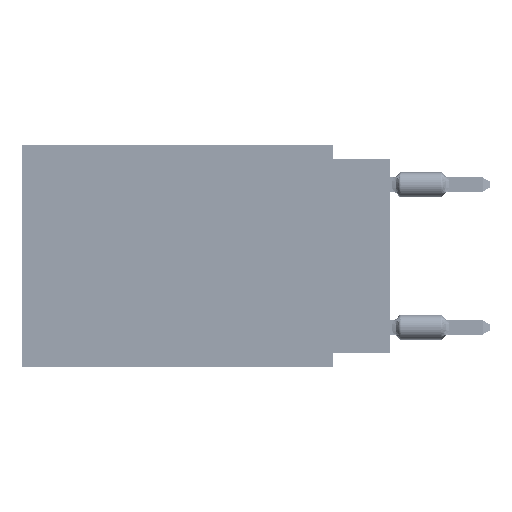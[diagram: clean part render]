
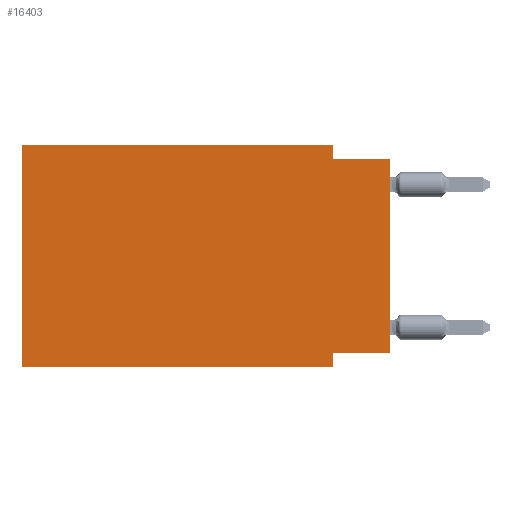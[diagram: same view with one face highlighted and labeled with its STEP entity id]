
A CAD part, left-side view. The second image highlights one B-rep face of the part: STEP entity #16403.
In plain terms, the highlighted planar face has unit normal (-1, 0, 0).
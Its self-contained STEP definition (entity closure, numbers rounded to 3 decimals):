
#2498 = PLANE ( 'NONE',  #29205 ) ;
#3460 = CARTESIAN_POINT ( 'NONE',  ( 0., 16.383, 0. ) ) ;
#4499 = DIRECTION ( 'NONE',  ( 0., 0., 1. ) ) ;
#5899 = ORIENTED_EDGE ( 'NONE', *, *, #72628, .F. ) ;
#9023 = CARTESIAN_POINT ( 'NONE',  ( 0., 16.383, 0. ) ) ;
#9397 = CARTESIAN_POINT ( 'NONE',  ( 0., 16.383, -9.906 ) ) ;
#9549 = VECTOR ( 'NONE', #66764, 1000. ) ;
#11398 = EDGE_CURVE ( 'NONE', #43634, #59774, #83114, .T. ) ;
#12213 = CARTESIAN_POINT ( 'NONE',  ( 0., 2.54, -0.635 ) ) ;
#13168 = VERTEX_POINT ( 'NONE', #40027 ) ;
#15576 = CARTESIAN_POINT ( 'NONE',  ( 0., 16.383, 0. ) ) ;
#15916 = LINE ( 'NONE', #9397, #35079 ) ;
#16403 = ADVANCED_FACE ( 'NONE', ( #55462 ), #2498, .F. ) ;
#19029 = LINE ( 'NONE', #39016, #73294 ) ;
#19997 = VECTOR ( 'NONE', #4499, 1000. ) ;
#20583 = DIRECTION ( 'NONE',  ( 0., 0., -1. ) ) ;
#21373 = VECTOR ( 'NONE', #48585, 1000. ) ;
#24513 = VERTEX_POINT ( 'NONE', #62157 ) ;
#25039 = CARTESIAN_POINT ( 'NONE',  ( 0., 0., -9.271 ) ) ;
#25801 = LINE ( 'NONE', #33173, #53826 ) ;
#26759 = EDGE_CURVE ( 'NONE', #47627, #76217, #25801, .T. ) ;
#27431 = ORIENTED_EDGE ( 'NONE', *, *, #43251, .F. ) ;
#29205 = AXIS2_PLACEMENT_3D ( 'NONE', #9023, #81532, #74999 ) ;
#29283 = VECTOR ( 'NONE', #32842, 1000. ) ;
#30302 = VERTEX_POINT ( 'NONE', #3460 ) ;
#30586 = VECTOR ( 'NONE', #82676, 1000. ) ;
#32842 = DIRECTION ( 'NONE',  ( 0., 1., 0. ) ) ;
#33161 = EDGE_CURVE ( 'NONE', #43634, #47627, #64108, .T. ) ;
#33173 = CARTESIAN_POINT ( 'NONE',  ( 0., 2.54, -9.906 ) ) ;
#34630 = LINE ( 'NONE', #47665, #9549 ) ;
#35079 = VECTOR ( 'NONE', #49338, 1000. ) ;
#36325 = EDGE_CURVE ( 'NONE', #24513, #30302, #56588, .T. ) ;
#37360 = CARTESIAN_POINT ( 'NONE',  ( 0., 2.54, -9.906 ) ) ;
#39016 = CARTESIAN_POINT ( 'NONE',  ( 0., 2.54, 0. ) ) ;
#39437 = DIRECTION ( 'NONE',  ( 0., 0., -1. ) ) ;
#39905 = ORIENTED_EDGE ( 'NONE', *, *, #33161, .F. ) ;
#40027 = CARTESIAN_POINT ( 'NONE',  ( 0., 2.54, 0. ) ) ;
#42087 = ORIENTED_EDGE ( 'NONE', *, *, #11398, .T. ) ;
#43251 = EDGE_CURVE ( 'NONE', #13168, #81314, #19029, .T. ) ;
#43634 = VERTEX_POINT ( 'NONE', #80858 ) ;
#46042 = ORIENTED_EDGE ( 'NONE', *, *, #36325, .F. ) ;
#47627 = VERTEX_POINT ( 'NONE', #64874 ) ;
#47665 = CARTESIAN_POINT ( 'NONE',  ( 0., 0., -0.635 ) ) ;
#48585 = DIRECTION ( 'NONE',  ( 0., -1., 0. ) ) ;
#49338 = DIRECTION ( 'NONE',  ( 0., -1., 0. ) ) ;
#50075 = EDGE_LOOP ( 'NONE', ( #42087, #5899, #27431, #53483, #46042, #65114, #59470, #39905 ) ) ;
#53483 = ORIENTED_EDGE ( 'NONE', *, *, #66517, .F. ) ;
#53826 = VECTOR ( 'NONE', #20583, 1000. ) ;
#55462 = FACE_OUTER_BOUND ( 'NONE', #50075, .T. ) ;
#56184 = CARTESIAN_POINT ( 'NONE',  ( 0., 0., 0. ) ) ;
#56588 = LINE ( 'NONE', #82651, #19997 ) ;
#59470 = ORIENTED_EDGE ( 'NONE', *, *, #26759, .F. ) ;
#59774 = VERTEX_POINT ( 'NONE', #79461 ) ;
#62157 = CARTESIAN_POINT ( 'NONE',  ( 0., 16.383, -9.906 ) ) ;
#64108 = LINE ( 'NONE', #25039, #29283 ) ;
#64874 = CARTESIAN_POINT ( 'NONE',  ( 0., 2.54, -9.271 ) ) ;
#65114 = ORIENTED_EDGE ( 'NONE', *, *, #79131, .T. ) ;
#66517 = EDGE_CURVE ( 'NONE', #30302, #13168, #68119, .T. ) ;
#66764 = DIRECTION ( 'NONE',  ( 0., -1., 0. ) ) ;
#68119 = LINE ( 'NONE', #15576, #21373 ) ;
#72628 = EDGE_CURVE ( 'NONE', #81314, #59774, #34630, .T. ) ;
#73294 = VECTOR ( 'NONE', #39437, 1000. ) ;
#74999 = DIRECTION ( 'NONE',  ( 0., 0., -1. ) ) ;
#76217 = VERTEX_POINT ( 'NONE', #37360 ) ;
#79131 = EDGE_CURVE ( 'NONE', #24513, #76217, #15916, .T. ) ;
#79461 = CARTESIAN_POINT ( 'NONE',  ( 0., 0., -0.635 ) ) ;
#80858 = CARTESIAN_POINT ( 'NONE',  ( 0., 0., -9.271 ) ) ;
#81314 = VERTEX_POINT ( 'NONE', #12213 ) ;
#81532 = DIRECTION ( 'NONE',  ( 1., 0., 0. ) ) ;
#82651 = CARTESIAN_POINT ( 'NONE',  ( 0., 16.383, 0. ) ) ;
#82676 = DIRECTION ( 'NONE',  ( 0., 0., 1. ) ) ;
#83114 = LINE ( 'NONE', #56184, #30586 ) ;
